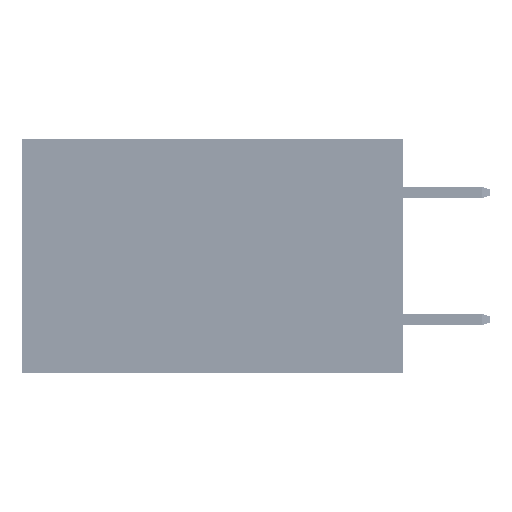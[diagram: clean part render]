
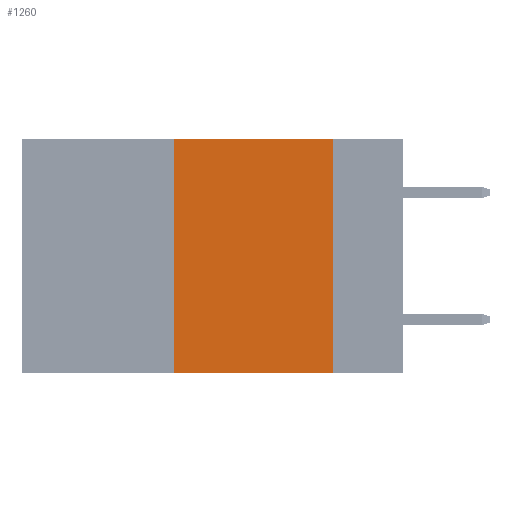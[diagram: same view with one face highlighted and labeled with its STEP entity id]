
A CAD part, left-side view. The second image highlights one B-rep face of the part: STEP entity #1260.
In plain terms, the highlighted planar face has unit normal (-1, 0, 0).
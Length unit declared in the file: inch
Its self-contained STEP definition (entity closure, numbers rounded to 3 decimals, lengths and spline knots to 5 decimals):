
#1260 = ADVANCED_FACE ( 'NONE', ( #38668 ), #11439, .F. ) ;
#2516 = EDGE_CURVE ( 'NONE', #42349, #26664, #49023, .T. ) ;
#3181 = VECTOR ( 'NONE', #40670, 39.37008 ) ;
#4638 = CARTESIAN_POINT ( 'NONE',  ( 0., 0.6, -0.37 ) ) ;
#5206 = VECTOR ( 'NONE', #35998, 39.37008 ) ;
#5320 = ORIENTED_EDGE ( 'NONE', *, *, #31801, .F. ) ;
#5585 = CARTESIAN_POINT ( 'NONE',  ( 0., 0.11, -0.37 ) ) ;
#6315 = DIRECTION ( 'NONE',  ( 0., 0., -1. ) ) ;
#8801 = LINE ( 'NONE', #28630, #3181 ) ;
#11439 = PLANE ( 'NONE',  #34193 ) ;
#12045 = CARTESIAN_POINT ( 'NONE',  ( 0., 0.36, 0. ) ) ;
#20066 = LINE ( 'NONE', #12045, #29857 ) ;
#21305 = CARTESIAN_POINT ( 'NONE',  ( 0., 0.11, 0. ) ) ;
#22898 = DIRECTION ( 'NONE',  ( 0., 0., 1. ) ) ;
#23587 = VECTOR ( 'NONE', #40278, 39.37008 ) ;
#23911 = CARTESIAN_POINT ( 'NONE',  ( 0., 0.36, 0. ) ) ;
#25112 = ORIENTED_EDGE ( 'NONE', *, *, #40736, .T. ) ;
#26255 = CARTESIAN_POINT ( 'NONE',  ( 0., 0.11, 0. ) ) ;
#26664 = VERTEX_POINT ( 'NONE', #5585 ) ;
#27437 = VERTEX_POINT ( 'NONE', #31741 ) ;
#28630 = CARTESIAN_POINT ( 'NONE',  ( 0., 0.6, 0. ) ) ;
#29857 = VECTOR ( 'NONE', #22898, 39.37008 ) ;
#31741 = CARTESIAN_POINT ( 'NONE',  ( 0., 0.36, -0.37 ) ) ;
#31801 = EDGE_CURVE ( 'NONE', #27437, #42661, #20066, .T. ) ;
#33250 = EDGE_LOOP ( 'NONE', ( #42040, #42104, #5320, #25112 ) ) ;
#34193 = AXIS2_PLACEMENT_3D ( 'NONE', #50506, #46155, #6315 ) ;
#35998 = DIRECTION ( 'NONE',  ( 0., -1., 0. ) ) ;
#37831 = EDGE_CURVE ( 'NONE', #42661, #42349, #8801, .T. ) ;
#38668 = FACE_OUTER_BOUND ( 'NONE', #33250, .T. ) ;
#40278 = DIRECTION ( 'NONE',  ( 0., 0., -1. ) ) ;
#40670 = DIRECTION ( 'NONE',  ( 0., -1., 0. ) ) ;
#40736 = EDGE_CURVE ( 'NONE', #27437, #26664, #43690, .T. ) ;
#42040 = ORIENTED_EDGE ( 'NONE', *, *, #2516, .F. ) ;
#42104 = ORIENTED_EDGE ( 'NONE', *, *, #37831, .F. ) ;
#42349 = VERTEX_POINT ( 'NONE', #26255 ) ;
#42661 = VERTEX_POINT ( 'NONE', #23911 ) ;
#43690 = LINE ( 'NONE', #4638, #5206 ) ;
#46155 = DIRECTION ( 'NONE',  ( 1., 0., 0. ) ) ;
#49023 = LINE ( 'NONE', #21305, #23587 ) ;
#50506 = CARTESIAN_POINT ( 'NONE',  ( 0., 0.6, 0. ) ) ;
